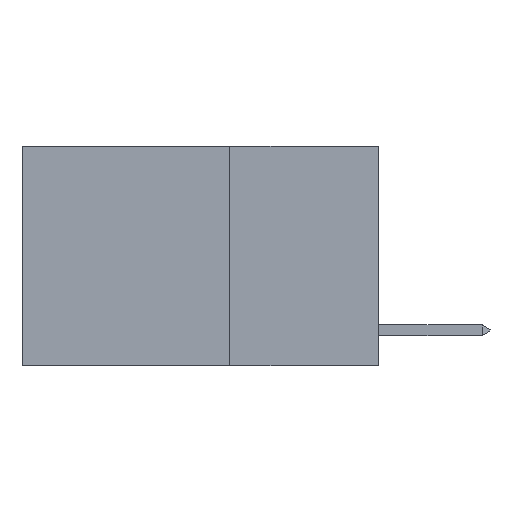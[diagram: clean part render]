
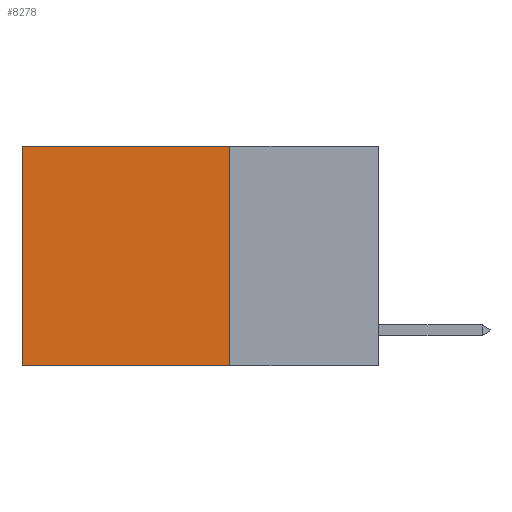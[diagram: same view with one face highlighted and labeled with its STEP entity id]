
A CAD part, left-side view. The second image highlights one B-rep face of the part: STEP entity #8278.
In plain terms, the highlighted planar face has unit normal (-1, 0, 0).
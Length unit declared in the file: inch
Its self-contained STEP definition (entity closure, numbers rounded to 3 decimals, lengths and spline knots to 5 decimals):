
#158 = AXIS2_PLACEMENT_3D ( 'NONE', #8514, #4079, #6993 ) ;
#184 = CARTESIAN_POINT ( 'NONE',  ( 0.2625, 0.25, 0. ) ) ;
#239 = CARTESIAN_POINT ( 'NONE',  ( 0.2625, 0.25, 0. ) ) ;
#246 = EDGE_CURVE ( 'NONE', #1704, #4744, #3714, .T. ) ;
#773 = VECTOR ( 'NONE', #5605, 39.37008 ) ;
#785 = DIRECTION ( 'NONE',  ( 0., 1., 0. ) ) ;
#983 = EDGE_CURVE ( 'NONE', #5180, #9533, #4188, .T. ) ;
#1704 = VERTEX_POINT ( 'NONE', #3166 ) ;
#1928 = EDGE_CURVE ( 'NONE', #9533, #4744, #5532, .T. ) ;
#1930 = PLANE ( 'NONE',  #158 ) ;
#2416 = CARTESIAN_POINT ( 'NONE',  ( 0.2625, 0.25, -0.37 ) ) ;
#2453 = VECTOR ( 'NONE', #8316, 39.37008 ) ;
#2752 = CARTESIAN_POINT ( 'NONE',  ( 0.2625, 0.25, 0. ) ) ;
#3166 = CARTESIAN_POINT ( 'NONE',  ( 0.2625, 0.25, -0.37 ) ) ;
#3714 = LINE ( 'NONE', #2416, #7132 ) ;
#3842 = ORIENTED_EDGE ( 'NONE', *, *, #1928, .T. ) ;
#4079 = DIRECTION ( 'NONE',  ( 1., 0., 0. ) ) ;
#4188 = LINE ( 'NONE', #2752, #773 ) ;
#4215 = CARTESIAN_POINT ( 'NONE',  ( 0.2625, 0.6, 0. ) ) ;
#4744 = VERTEX_POINT ( 'NONE', #8567 ) ;
#5180 = VERTEX_POINT ( 'NONE', #239 ) ;
#5439 = ORIENTED_EDGE ( 'NONE', *, *, #246, .F. ) ;
#5532 = LINE ( 'NONE', #4215, #8409 ) ;
#5589 = FACE_OUTER_BOUND ( 'NONE', #6669, .T. ) ;
#5605 = DIRECTION ( 'NONE',  ( 0., 1., 0. ) ) ;
#6669 = EDGE_LOOP ( 'NONE', ( #3842, #5439, #8706, #9377 ) ) ;
#6693 = LINE ( 'NONE', #184, #2453 ) ;
#6993 = DIRECTION ( 'NONE',  ( 0., 0., -1. ) ) ;
#7022 = DIRECTION ( 'NONE',  ( 0., 0., -1. ) ) ;
#7132 = VECTOR ( 'NONE', #785, 39.37008 ) ;
#7769 = CARTESIAN_POINT ( 'NONE',  ( 0.2625, 0.6, 0. ) ) ;
#8278 = ADVANCED_FACE ( 'NONE', ( #5589 ), #1930, .F. ) ;
#8316 = DIRECTION ( 'NONE',  ( 0., 0., -1. ) ) ;
#8409 = VECTOR ( 'NONE', #7022, 39.37008 ) ;
#8514 = CARTESIAN_POINT ( 'NONE',  ( 0.2625, 0.25, 0. ) ) ;
#8551 = EDGE_CURVE ( 'NONE', #5180, #1704, #6693, .T. ) ;
#8567 = CARTESIAN_POINT ( 'NONE',  ( 0.2625, 0.6, -0.37 ) ) ;
#8706 = ORIENTED_EDGE ( 'NONE', *, *, #8551, .F. ) ;
#9377 = ORIENTED_EDGE ( 'NONE', *, *, #983, .T. ) ;
#9533 = VERTEX_POINT ( 'NONE', #7769 ) ;
